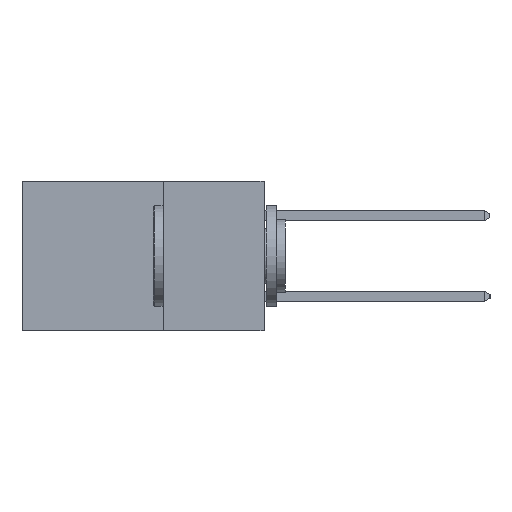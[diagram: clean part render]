
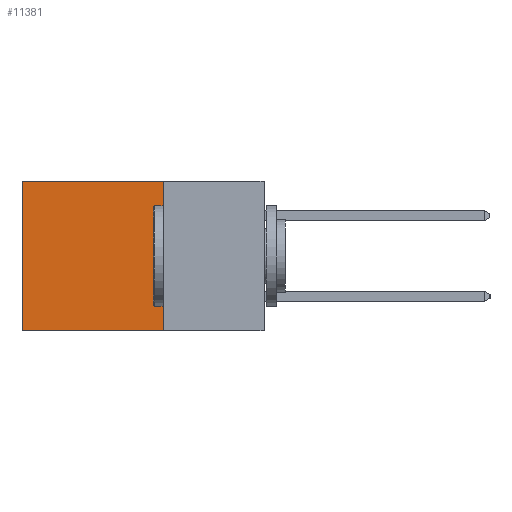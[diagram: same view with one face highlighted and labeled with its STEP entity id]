
A CAD part, left-side view. The second image highlights one B-rep face of the part: STEP entity #11381.
In plain terms, the highlighted planar face has unit normal (-1, 0, 0).
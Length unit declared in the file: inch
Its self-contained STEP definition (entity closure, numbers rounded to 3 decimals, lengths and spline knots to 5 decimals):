
#837 = ORIENTED_EDGE ( 'NONE', *, *, #9974, .F. ) ;
#2786 = VERTEX_POINT ( 'NONE', #6424 ) ;
#3195 = VERTEX_POINT ( 'NONE', #3366 ) ;
#3366 = CARTESIAN_POINT ( 'NONE',  ( 0.2615, 0.25, 0. ) ) ;
#3375 = EDGE_CURVE ( 'NONE', #3195, #12720, #13224, .T. ) ;
#3479 = AXIS2_PLACEMENT_3D ( 'NONE', #13457, #7435, #15487 ) ;
#4317 = EDGE_CURVE ( 'NONE', #12720, #5593, #11323, .T. ) ;
#4347 = CARTESIAN_POINT ( 'NONE',  ( 0.2615, 0.6, -0.37 ) ) ;
#4857 = DIRECTION ( 'NONE',  ( 0., 1., 0. ) ) ;
#5104 = EDGE_CURVE ( 'NONE', #2786, #5593, #12050, .T. ) ;
#5593 = VERTEX_POINT ( 'NONE', #15206 ) ;
#5791 = CARTESIAN_POINT ( 'NONE',  ( 0.2615, 0.25, -0.37 ) ) ;
#5844 = DIRECTION ( 'NONE',  ( 0., 0., -1. ) ) ;
#6218 = PLANE ( 'NONE',  #3479 ) ;
#6424 = CARTESIAN_POINT ( 'NONE',  ( 0.2615, 0.25, -0.37 ) ) ;
#6597 = CARTESIAN_POINT ( 'NONE',  ( 0.2615, 0.6, 0. ) ) ;
#7180 = VECTOR ( 'NONE', #4857, 39.37008 ) ;
#7435 = DIRECTION ( 'NONE',  ( 1., 0., 0. ) ) ;
#7776 = VECTOR ( 'NONE', #12821, 39.37008 ) ;
#9613 = CARTESIAN_POINT ( 'NONE',  ( 0.2615, 0.25, -0.37 ) ) ;
#9974 = EDGE_CURVE ( 'NONE', #3195, #2786, #15211, .T. ) ;
#10214 = ORIENTED_EDGE ( 'NONE', *, *, #5104, .F. ) ;
#10816 = DIRECTION ( 'NONE',  ( 0., 1., 0. ) ) ;
#11323 = LINE ( 'NONE', #4347, #7776 ) ;
#11381 = ADVANCED_FACE ( 'NONE', ( #11383 ), #6218, .F. ) ;
#11383 = FACE_OUTER_BOUND ( 'NONE', #14888, .T. ) ;
#11959 = VECTOR ( 'NONE', #5844, 39.37008 ) ;
#12029 = ORIENTED_EDGE ( 'NONE', *, *, #3375, .T. ) ;
#12050 = LINE ( 'NONE', #9613, #15293 ) ;
#12720 = VERTEX_POINT ( 'NONE', #6597 ) ;
#12821 = DIRECTION ( 'NONE',  ( 0., 0., -1. ) ) ;
#13224 = LINE ( 'NONE', #15763, #7180 ) ;
#13457 = CARTESIAN_POINT ( 'NONE',  ( 0.2615, 0.25, -0.37 ) ) ;
#13573 = ORIENTED_EDGE ( 'NONE', *, *, #4317, .T. ) ;
#14888 = EDGE_LOOP ( 'NONE', ( #13573, #10214, #837, #12029 ) ) ;
#15206 = CARTESIAN_POINT ( 'NONE',  ( 0.2615, 0.6, -0.37 ) ) ;
#15211 = LINE ( 'NONE', #5791, #11959 ) ;
#15293 = VECTOR ( 'NONE', #10816, 39.37008 ) ;
#15487 = DIRECTION ( 'NONE',  ( 0., 0., -1. ) ) ;
#15763 = CARTESIAN_POINT ( 'NONE',  ( 0.2615, 0.25, 0. ) ) ;
